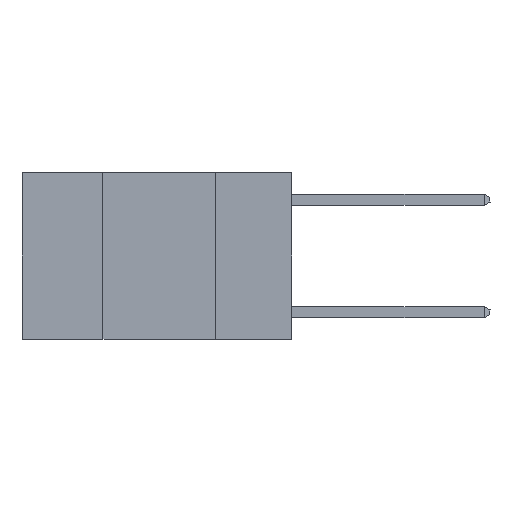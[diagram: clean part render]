
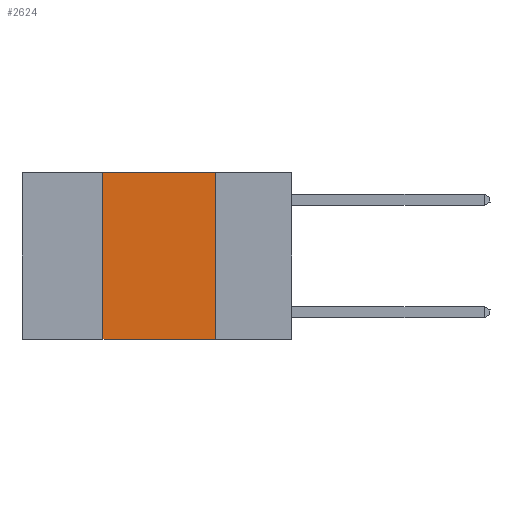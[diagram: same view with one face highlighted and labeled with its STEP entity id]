
A CAD part, left-side view. The second image highlights one B-rep face of the part: STEP entity #2624.
In plain terms, the highlighted planar face has unit normal (-1, 0, 0).
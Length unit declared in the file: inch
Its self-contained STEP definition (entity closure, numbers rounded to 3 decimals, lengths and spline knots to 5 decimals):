
#1628 = VECTOR ( 'NONE', #4532, 39.37008 ) ;
#1820 = EDGE_CURVE ( 'NONE', #4959, #7623, #6318, .T. ) ;
#1855 = CARTESIAN_POINT ( 'NONE',  ( 0., 0.6, -0.37 ) ) ;
#2624 = ADVANCED_FACE ( 'NONE', ( #7268 ), #4258, .F. ) ;
#2656 = CARTESIAN_POINT ( 'NONE',  ( 0., 0.17, 0. ) ) ;
#2967 = EDGE_CURVE ( 'NONE', #3888, #5914, #6637, .T. ) ;
#3142 = EDGE_LOOP ( 'NONE', ( #8401, #8079, #6043, #6463 ) ) ;
#3479 = CARTESIAN_POINT ( 'NONE',  ( 0., 0.6, 0. ) ) ;
#3502 = EDGE_CURVE ( 'NONE', #5914, #7623, #3543, .T. ) ;
#3543 = LINE ( 'NONE', #5912, #1628 ) ;
#3613 = VECTOR ( 'NONE', #4618, 39.37008 ) ;
#3888 = VERTEX_POINT ( 'NONE', #5230 ) ;
#4083 = CARTESIAN_POINT ( 'NONE',  ( 0., 0.42, -0.37 ) ) ;
#4258 = PLANE ( 'NONE',  #4909 ) ;
#4489 = VECTOR ( 'NONE', #8053, 39.37008 ) ;
#4532 = DIRECTION ( 'NONE',  ( 0., 0., -1. ) ) ;
#4618 = DIRECTION ( 'NONE',  ( 0., 0., 1. ) ) ;
#4909 = AXIS2_PLACEMENT_3D ( 'NONE', #5228, #7815, #7474 ) ;
#4959 = VERTEX_POINT ( 'NONE', #4083 ) ;
#5228 = CARTESIAN_POINT ( 'NONE',  ( 0., 0.6, 0. ) ) ;
#5230 = CARTESIAN_POINT ( 'NONE',  ( 0., 0.42, 0. ) ) ;
#5519 = LINE ( 'NONE', #5972, #3613 ) ;
#5710 = CARTESIAN_POINT ( 'NONE',  ( 0., 0.17, -0.37 ) ) ;
#5912 = CARTESIAN_POINT ( 'NONE',  ( 0., 0.17, 0. ) ) ;
#5914 = VERTEX_POINT ( 'NONE', #2656 ) ;
#5972 = CARTESIAN_POINT ( 'NONE',  ( 0., 0.42, 0. ) ) ;
#6043 = ORIENTED_EDGE ( 'NONE', *, *, #7975, .F. ) ;
#6318 = LINE ( 'NONE', #1855, #4489 ) ;
#6422 = VECTOR ( 'NONE', #8599, 39.37008 ) ;
#6463 = ORIENTED_EDGE ( 'NONE', *, *, #1820, .T. ) ;
#6637 = LINE ( 'NONE', #3479, #6422 ) ;
#7268 = FACE_OUTER_BOUND ( 'NONE', #3142, .T. ) ;
#7474 = DIRECTION ( 'NONE',  ( 0., 0., -1. ) ) ;
#7623 = VERTEX_POINT ( 'NONE', #5710 ) ;
#7815 = DIRECTION ( 'NONE',  ( 1., 0., 0. ) ) ;
#7975 = EDGE_CURVE ( 'NONE', #4959, #3888, #5519, .T. ) ;
#8053 = DIRECTION ( 'NONE',  ( 0., -1., 0. ) ) ;
#8079 = ORIENTED_EDGE ( 'NONE', *, *, #2967, .F. ) ;
#8401 = ORIENTED_EDGE ( 'NONE', *, *, #3502, .F. ) ;
#8599 = DIRECTION ( 'NONE',  ( 0., -1., 0. ) ) ;
